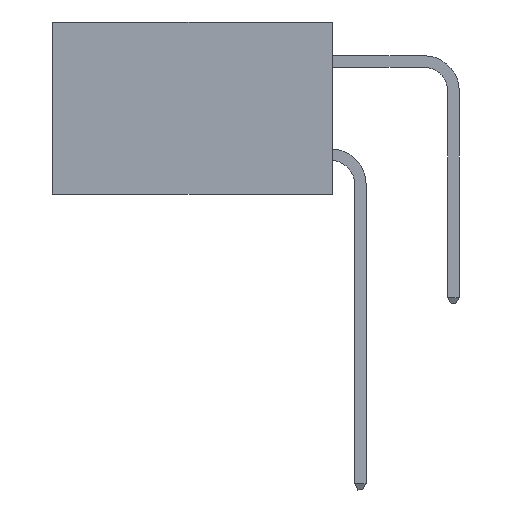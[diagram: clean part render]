
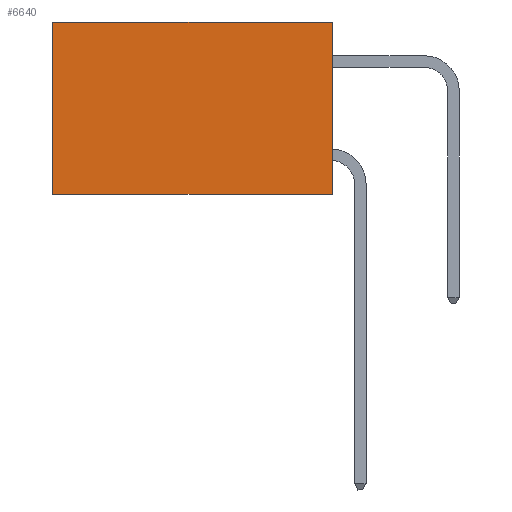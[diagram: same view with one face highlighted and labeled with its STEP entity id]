
A CAD part, left-side view. The second image highlights one B-rep face of the part: STEP entity #6640.
In plain terms, the highlighted planar face has unit normal (-1, 0, 0).
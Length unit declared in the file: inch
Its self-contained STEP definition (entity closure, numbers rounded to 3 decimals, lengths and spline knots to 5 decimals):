
#505 = DIRECTION ( 'NONE',  ( 0., 0., -1. ) ) ;
#2688 = CARTESIAN_POINT ( 'NONE',  ( 0.2615, 0.6, -0.37 ) ) ;
#2934 = EDGE_LOOP ( 'NONE', ( #15530, #19958, #21715, #20279 ) ) ;
#3681 = VECTOR ( 'NONE', #4996, 39.37008 ) ;
#4248 = EDGE_CURVE ( 'NONE', #22182, #22691, #9497, .T. ) ;
#4448 = EDGE_CURVE ( 'NONE', #17511, #22182, #19992, .T. ) ;
#4577 = VECTOR ( 'NONE', #11599, 39.37008 ) ;
#4996 = DIRECTION ( 'NONE',  ( 0., 1., 0. ) ) ;
#6088 = AXIS2_PLACEMENT_3D ( 'NONE', #23628, #12273, #505 ) ;
#6640 = ADVANCED_FACE ( 'NONE', ( #18247 ), #23213, .F. ) ;
#6739 = CARTESIAN_POINT ( 'NONE',  ( 0.2615, 0., 0. ) ) ;
#6808 = EDGE_CURVE ( 'NONE', #12832, #22691, #9510, .T. ) ;
#9110 = DIRECTION ( 'NONE',  ( 0., 0., -1. ) ) ;
#9497 = LINE ( 'NONE', #22410, #19117 ) ;
#9510 = LINE ( 'NONE', #10804, #3681 ) ;
#9622 = CARTESIAN_POINT ( 'NONE',  ( 0.2615, 0., 0. ) ) ;
#10804 = CARTESIAN_POINT ( 'NONE',  ( 0.2615, 0., -0.37 ) ) ;
#11599 = DIRECTION ( 'NONE',  ( 0., 1., 0. ) ) ;
#12273 = DIRECTION ( 'NONE',  ( 1., 0., 0. ) ) ;
#12832 = VERTEX_POINT ( 'NONE', #17999 ) ;
#12959 = DIRECTION ( 'NONE',  ( 0., 0., -1. ) ) ;
#13517 = LINE ( 'NONE', #14908, #19182 ) ;
#14908 = CARTESIAN_POINT ( 'NONE',  ( 0.2615, 0., -0.37 ) ) ;
#15530 = ORIENTED_EDGE ( 'NONE', *, *, #4248, .T. ) ;
#17511 = VERTEX_POINT ( 'NONE', #6739 ) ;
#17654 = EDGE_CURVE ( 'NONE', #17511, #12832, #13517, .T. ) ;
#17999 = CARTESIAN_POINT ( 'NONE',  ( 0.2615, 0., -0.37 ) ) ;
#18247 = FACE_OUTER_BOUND ( 'NONE', #2934, .T. ) ;
#18393 = CARTESIAN_POINT ( 'NONE',  ( 0.2615, 0.6, 0. ) ) ;
#19117 = VECTOR ( 'NONE', #12959, 39.37008 ) ;
#19182 = VECTOR ( 'NONE', #9110, 39.37008 ) ;
#19958 = ORIENTED_EDGE ( 'NONE', *, *, #6808, .F. ) ;
#19992 = LINE ( 'NONE', #9622, #4577 ) ;
#20279 = ORIENTED_EDGE ( 'NONE', *, *, #4448, .T. ) ;
#21715 = ORIENTED_EDGE ( 'NONE', *, *, #17654, .F. ) ;
#22182 = VERTEX_POINT ( 'NONE', #18393 ) ;
#22410 = CARTESIAN_POINT ( 'NONE',  ( 0.2615, 0.6, -0.37 ) ) ;
#22691 = VERTEX_POINT ( 'NONE', #2688 ) ;
#23213 = PLANE ( 'NONE',  #6088 ) ;
#23628 = CARTESIAN_POINT ( 'NONE',  ( 0.2615, 0., -0.37 ) ) ;
